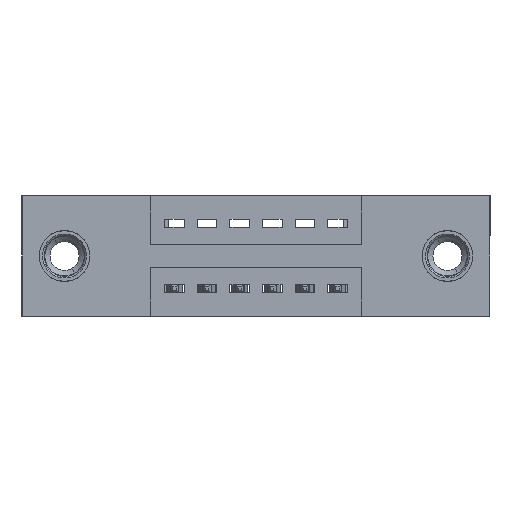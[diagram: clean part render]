
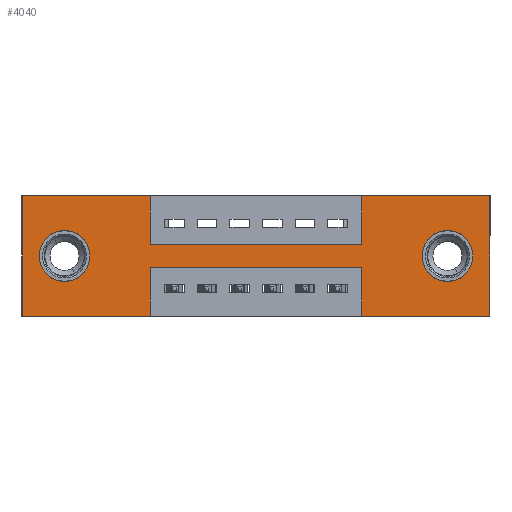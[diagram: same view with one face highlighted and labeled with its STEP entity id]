
A CAD part, front view. The second image highlights one B-rep face of the part: STEP entity #4040.
In plain terms, the highlighted planar face has unit normal (0, -1, 0).
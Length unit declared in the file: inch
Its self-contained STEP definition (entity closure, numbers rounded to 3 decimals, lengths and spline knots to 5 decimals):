
#26 = DIRECTION ( 'NONE',  ( 0., 0., -1. ) ) ;
#75 = CARTESIAN_POINT ( 'NONE',  ( 0., 0., -0.37 ) ) ;
#105 = VECTOR ( 'NONE', #2294, 39.37008 ) ;
#595 = DIRECTION ( 'NONE',  ( 1., 0., 0. ) ) ;
#649 = LINE ( 'NONE', #7614, #105 ) ;
#673 = CARTESIAN_POINT ( 'NONE',  ( 1.0425, 0., 0. ) ) ;
#761 = VERTEX_POINT ( 'NONE', #7730 ) ;
#894 = VECTOR ( 'NONE', #4643, 39.37008 ) ;
#914 = CARTESIAN_POINT ( 'NONE',  ( 0.13, 0., -0.107 ) ) ;
#1066 = DIRECTION ( 'NONE',  ( 1., 0., 0. ) ) ;
#1110 = ORIENTED_EDGE ( 'NONE', *, *, #3804, .F. ) ;
#1121 = FACE_BOUND ( 'NONE', #5803, .T. ) ;
#1133 = LINE ( 'NONE', #4075, #10338 ) ;
#1307 = DIRECTION ( 'NONE',  ( 0., 1., 0. ) ) ;
#1335 = CIRCLE ( 'NONE', #3838, 0.078 ) ;
#1460 = EDGE_CURVE ( 'NONE', #761, #6288, #10402, .T. ) ;
#1489 = CARTESIAN_POINT ( 'NONE',  ( 0., 0., 0. ) ) ;
#1600 = CARTESIAN_POINT ( 'NONE',  ( 0.13, 0., -0.185 ) ) ;
#1653 = PLANE ( 'NONE',  #8366 ) ;
#1774 = VECTOR ( 'NONE', #9790, 39.37008 ) ;
#1818 = VERTEX_POINT ( 'NONE', #10463 ) ;
#1822 = EDGE_CURVE ( 'NONE', #10499, #10556, #6354, .T. ) ;
#1872 = CARTESIAN_POINT ( 'NONE',  ( 0.3925, 0., -0.15 ) ) ;
#1950 = ORIENTED_EDGE ( 'NONE', *, *, #1460, .F. ) ;
#2004 = EDGE_CURVE ( 'NONE', #4022, #6316, #7597, .T. ) ;
#2093 = VERTEX_POINT ( 'NONE', #4479 ) ;
#2214 = EDGE_CURVE ( 'NONE', #5746, #4315, #8177, .T. ) ;
#2252 = DIRECTION ( 'NONE',  ( 0., 0., 1. ) ) ;
#2294 = DIRECTION ( 'NONE',  ( 0., 0., -1. ) ) ;
#2317 = CARTESIAN_POINT ( 'NONE',  ( 1.305, 0., -0.185 ) ) ;
#2333 = ORIENTED_EDGE ( 'NONE', *, *, #3353, .F. ) ;
#2428 = DIRECTION ( 'NONE',  ( 0., 0., 1. ) ) ;
#2583 = CARTESIAN_POINT ( 'NONE',  ( 1.0425, 0., -0.37 ) ) ;
#2765 = DIRECTION ( 'NONE',  ( 0., 0., -1. ) ) ;
#2777 = EDGE_CURVE ( 'NONE', #4201, #2093, #4820, .T. ) ;
#2873 = LINE ( 'NONE', #7534, #3566 ) ;
#2895 = CARTESIAN_POINT ( 'NONE',  ( 1.305, 0., -0.185 ) ) ;
#2974 = CARTESIAN_POINT ( 'NONE',  ( 1.0425, 0., -0.22 ) ) ;
#3106 = VERTEX_POINT ( 'NONE', #10356 ) ;
#3153 = ORIENTED_EDGE ( 'NONE', *, *, #1822, .F. ) ;
#3202 = VERTEX_POINT ( 'NONE', #5964 ) ;
#3217 = LINE ( 'NONE', #3389, #10601 ) ;
#3353 = EDGE_CURVE ( 'NONE', #3202, #1818, #8888, .T. ) ;
#3389 = CARTESIAN_POINT ( 'NONE',  ( 1.0425, 0., 0. ) ) ;
#3415 = CARTESIAN_POINT ( 'NONE',  ( 0.13, 0., -0.185 ) ) ;
#3489 = DIRECTION ( 'NONE',  ( 0., 1., 0. ) ) ;
#3566 = VECTOR ( 'NONE', #2252, 39.37008 ) ;
#3804 = EDGE_CURVE ( 'NONE', #1818, #10499, #3217, .T. ) ;
#3810 = DIRECTION ( 'NONE',  ( 0., 0., -1. ) ) ;
#3838 = AXIS2_PLACEMENT_3D ( 'NONE', #2317, #1307, #26 ) ;
#4022 = VERTEX_POINT ( 'NONE', #914 ) ;
#4040 = ADVANCED_FACE ( 'NONE', ( #1121, #10072, #9230 ), #1653, .T. ) ;
#4075 = CARTESIAN_POINT ( 'NONE',  ( 1.435, 0., 0. ) ) ;
#4201 = VERTEX_POINT ( 'NONE', #4758 ) ;
#4204 = DIRECTION ( 'NONE',  ( -1., 0., 0. ) ) ;
#4315 = VERTEX_POINT ( 'NONE', #11277 ) ;
#4359 = DIRECTION ( 'NONE',  ( 0., 0., 1. ) ) ;
#4406 = CARTESIAN_POINT ( 'NONE',  ( 0.13, 0., -0.263 ) ) ;
#4479 = CARTESIAN_POINT ( 'NONE',  ( 0.3925, 0., -0.37 ) ) ;
#4488 = AXIS2_PLACEMENT_3D ( 'NONE', #3415, #3489, #10612 ) ;
#4643 = DIRECTION ( 'NONE',  ( 1., 0., 0. ) ) ;
#4758 = CARTESIAN_POINT ( 'NONE',  ( 0.3925, 0., -0.22 ) ) ;
#4820 = LINE ( 'NONE', #8112, #11350 ) ;
#4920 = AXIS2_PLACEMENT_3D ( 'NONE', #2895, #9193, #3810 ) ;
#5056 = VECTOR ( 'NONE', #4204, 39.37008 ) ;
#5120 = DIRECTION ( 'NONE',  ( 0., 0., 1. ) ) ;
#5191 = DIRECTION ( 'NONE',  ( 0., 1., 0. ) ) ;
#5746 = VERTEX_POINT ( 'NONE', #11095 ) ;
#5803 = EDGE_LOOP ( 'NONE', ( #7832, #11052 ) ) ;
#5829 = EDGE_CURVE ( 'NONE', #4315, #5746, #1335, .T. ) ;
#5899 = DIRECTION ( 'NONE',  ( -1., 0., 0. ) ) ;
#5927 = ORIENTED_EDGE ( 'NONE', *, *, #2777, .F. ) ;
#5945 = LINE ( 'NONE', #6386, #7468 ) ;
#5964 = CARTESIAN_POINT ( 'NONE',  ( 0.3925, 0., -0.15 ) ) ;
#6009 = ORIENTED_EDGE ( 'NONE', *, *, #9695, .F. ) ;
#6288 = VERTEX_POINT ( 'NONE', #2583 ) ;
#6316 = VERTEX_POINT ( 'NONE', #4406 ) ;
#6354 = LINE ( 'NONE', #1489, #11230 ) ;
#6386 = CARTESIAN_POINT ( 'NONE',  ( 0., 0., 0. ) ) ;
#6390 = DIRECTION ( 'NONE',  ( 0., -1., 0. ) ) ;
#6444 = EDGE_CURVE ( 'NONE', #3106, #6838, #5945, .T. ) ;
#6567 = VERTEX_POINT ( 'NONE', #2974 ) ;
#6608 = EDGE_CURVE ( 'NONE', #6288, #6567, #2873, .T. ) ;
#6751 = LINE ( 'NONE', #11475, #9976 ) ;
#6838 = VERTEX_POINT ( 'NONE', #6856 ) ;
#6856 = CARTESIAN_POINT ( 'NONE',  ( 0.3925, 0., 0. ) ) ;
#7042 = CARTESIAN_POINT ( 'NONE',  ( 0., 0., -0.37 ) ) ;
#7067 = EDGE_CURVE ( 'NONE', #9659, #3106, #6751, .T. ) ;
#7293 = ORIENTED_EDGE ( 'NONE', *, *, #10008, .F. ) ;
#7357 = AXIS2_PLACEMENT_3D ( 'NONE', #1600, #5191, #5120 ) ;
#7420 = ORIENTED_EDGE ( 'NONE', *, *, #10903, .F. ) ;
#7468 = VECTOR ( 'NONE', #1066, 39.37008 ) ;
#7534 = CARTESIAN_POINT ( 'NONE',  ( 1.0425, 0., -0.37 ) ) ;
#7544 = ORIENTED_EDGE ( 'NONE', *, *, #6608, .F. ) ;
#7597 = CIRCLE ( 'NONE', #4488, 0.078 ) ;
#7614 = CARTESIAN_POINT ( 'NONE',  ( 0.3925, 0., 0. ) ) ;
#7730 = CARTESIAN_POINT ( 'NONE',  ( 1.435, 0., -0.37 ) ) ;
#7832 = ORIENTED_EDGE ( 'NONE', *, *, #2214, .T. ) ;
#7863 = CARTESIAN_POINT ( 'NONE',  ( 1.435, 0., 0. ) ) ;
#8112 = CARTESIAN_POINT ( 'NONE',  ( 0.3925, 0., -0.37 ) ) ;
#8177 = CIRCLE ( 'NONE', #4920, 0.078 ) ;
#8225 = EDGE_LOOP ( 'NONE', ( #5927, #8852, #7544, #1950, #6009, #3153, #1110, #2333, #7420, #9995, #8259, #7293 ) ) ;
#8259 = ORIENTED_EDGE ( 'NONE', *, *, #7067, .F. ) ;
#8366 = AXIS2_PLACEMENT_3D ( 'NONE', #7042, #6390, #10891 ) ;
#8376 = ORIENTED_EDGE ( 'NONE', *, *, #2004, .T. ) ;
#8384 = CARTESIAN_POINT ( 'NONE',  ( 0., 0., -0.37 ) ) ;
#8457 = VECTOR ( 'NONE', #5899, 39.37008 ) ;
#8508 = LINE ( 'NONE', #75, #1774 ) ;
#8721 = CARTESIAN_POINT ( 'NONE',  ( 0.3925, 0., -0.22 ) ) ;
#8852 = ORIENTED_EDGE ( 'NONE', *, *, #9225, .F. ) ;
#8888 = LINE ( 'NONE', #1872, #894 ) ;
#8975 = CIRCLE ( 'NONE', #7357, 0.078 ) ;
#9193 = DIRECTION ( 'NONE',  ( 0., 1., 0. ) ) ;
#9225 = EDGE_CURVE ( 'NONE', #6567, #4201, #9260, .T. ) ;
#9230 = FACE_OUTER_BOUND ( 'NONE', #8225, .T. ) ;
#9241 = EDGE_CURVE ( 'NONE', #6316, #4022, #8975, .T. ) ;
#9260 = LINE ( 'NONE', #8721, #5056 ) ;
#9659 = VERTEX_POINT ( 'NONE', #8384 ) ;
#9695 = EDGE_CURVE ( 'NONE', #10556, #761, #1133, .T. ) ;
#9790 = DIRECTION ( 'NONE',  ( -1., 0., 0. ) ) ;
#9976 = VECTOR ( 'NONE', #4359, 39.37008 ) ;
#9995 = ORIENTED_EDGE ( 'NONE', *, *, #6444, .F. ) ;
#10008 = EDGE_CURVE ( 'NONE', #2093, #9659, #8508, .T. ) ;
#10072 = FACE_BOUND ( 'NONE', #11428, .T. ) ;
#10338 = VECTOR ( 'NONE', #11266, 39.37008 ) ;
#10356 = CARTESIAN_POINT ( 'NONE',  ( 0., 0., 0. ) ) ;
#10369 = CARTESIAN_POINT ( 'NONE',  ( 0., 0., -0.37 ) ) ;
#10402 = LINE ( 'NONE', #10369, #8457 ) ;
#10463 = CARTESIAN_POINT ( 'NONE',  ( 1.0425, 0., -0.15 ) ) ;
#10473 = ORIENTED_EDGE ( 'NONE', *, *, #9241, .T. ) ;
#10499 = VERTEX_POINT ( 'NONE', #673 ) ;
#10556 = VERTEX_POINT ( 'NONE', #7863 ) ;
#10601 = VECTOR ( 'NONE', #2428, 39.37008 ) ;
#10612 = DIRECTION ( 'NONE',  ( 0., 0., 1. ) ) ;
#10891 = DIRECTION ( 'NONE',  ( 0., 0., -1. ) ) ;
#10903 = EDGE_CURVE ( 'NONE', #6838, #3202, #649, .T. ) ;
#11052 = ORIENTED_EDGE ( 'NONE', *, *, #5829, .T. ) ;
#11095 = CARTESIAN_POINT ( 'NONE',  ( 1.305, 0., -0.107 ) ) ;
#11230 = VECTOR ( 'NONE', #595, 39.37008 ) ;
#11266 = DIRECTION ( 'NONE',  ( 0., 0., -1. ) ) ;
#11277 = CARTESIAN_POINT ( 'NONE',  ( 1.305, 0., -0.263 ) ) ;
#11350 = VECTOR ( 'NONE', #2765, 39.37008 ) ;
#11428 = EDGE_LOOP ( 'NONE', ( #8376, #10473 ) ) ;
#11475 = CARTESIAN_POINT ( 'NONE',  ( 0., 0., 0. ) ) ;
